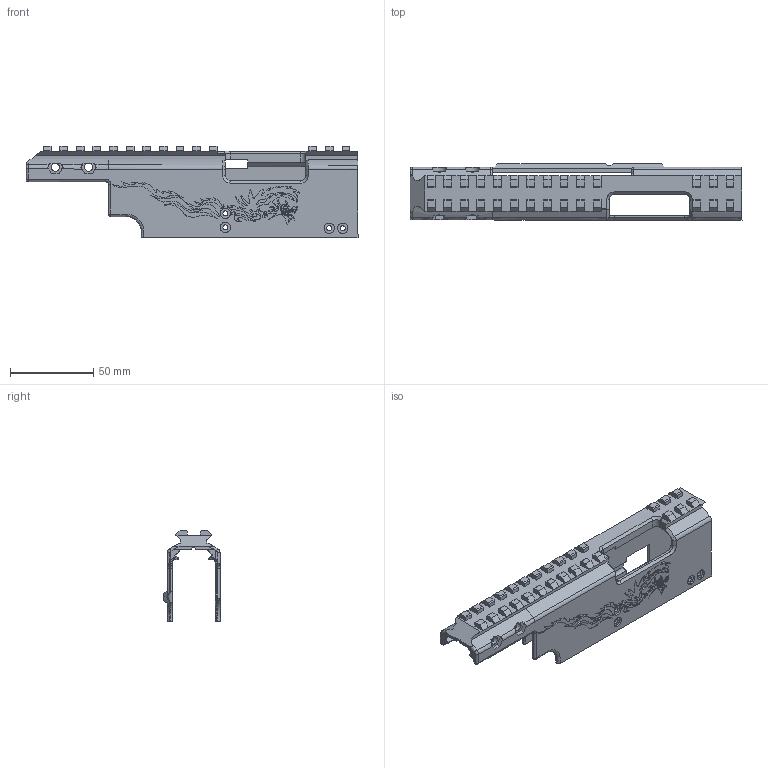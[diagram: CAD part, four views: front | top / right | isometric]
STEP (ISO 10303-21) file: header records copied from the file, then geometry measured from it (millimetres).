
FILE_DESCRIPTION(/* description */ (''),/* implementation_level */ '2;1');
FILE_NAME(/* name */ 'dust cover .step',/* time_stamp */ '2021-09-02T19:31:52-05:00',/* author */ (''),/* organization */ (''),/* preprocessor_version */ 'ST-DEVELOPER v18.1',/* originating_system */ 'Autodesk Translation Framework v10.10.0.1391',/* authorisation */ '');
FILE_SCHEMA (('AUTOMOTIVE_DESIGN { 1 0 10303 214 3 1 1 }'));
Products named in the file (1): dust cover primary
Bounding box: 199.9 x 33.8 x 54.91 mm (x, y, z)
Volume: 62141.3 mm3; surface area: 43305.8 mm2
Topology: 1 solids, 1 shells, 1572 faces, 4565 edges, 3017 vertices
Faces by surface type: bspline 1155, plane 338, cylinder 70, sphere 4, torus 4, cone 1
Full cylindrical faces by diameter (mm): 3 x8, 5 x4, 6.2 x8
Entity records: 57444 total; most frequent: CARTESIAN_POINT 26680, ORIENTED_EDGE 9120, EDGE_CURVE 4560, DIRECTION 3182, VERTEX_POINT 3016, LINE 2016, VECTOR 2016, EDGE_LOOP 1626
